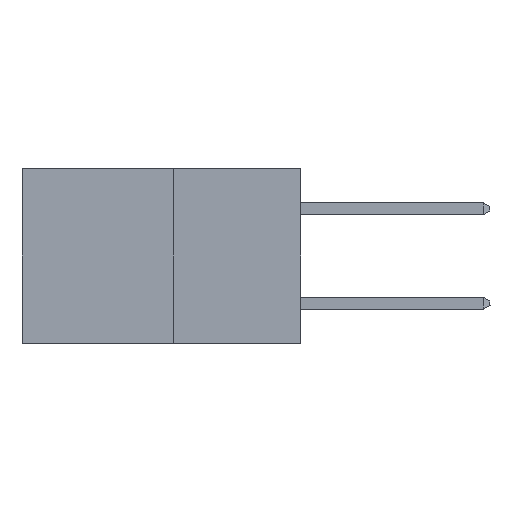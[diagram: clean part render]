
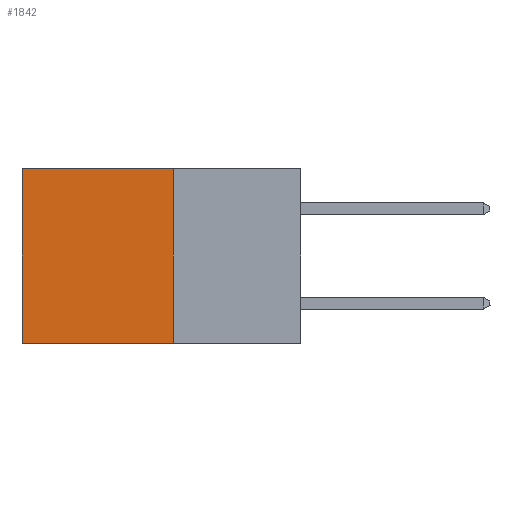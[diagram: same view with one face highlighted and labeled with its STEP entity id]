
A CAD part, left-side view. The second image highlights one B-rep face of the part: STEP entity #1842.
In plain terms, the highlighted planar face has unit normal (-1, 0, 0).
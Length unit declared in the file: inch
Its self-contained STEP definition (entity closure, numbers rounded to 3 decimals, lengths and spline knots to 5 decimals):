
#61 = CARTESIAN_POINT ( 'NONE',  ( 0.277, 0.27, -0.37 ) ) ;
#102 = CARTESIAN_POINT ( 'NONE',  ( 0.277, 0.27, -0.37 ) ) ;
#252 = DIRECTION ( 'NONE',  ( 0., 1., 0. ) ) ;
#1842 = ADVANCED_FACE ( 'NONE', ( #4763 ), #10210, .F. ) ;
#2571 = VERTEX_POINT ( 'NONE', #7368 ) ;
#2665 = EDGE_CURVE ( 'NONE', #8172, #17340, #2743, .T. ) ;
#2743 = LINE ( 'NONE', #9272, #13360 ) ;
#3216 = CARTESIAN_POINT ( 'NONE',  ( 0.277, 0.59, 0. ) ) ;
#4574 = DIRECTION ( 'NONE',  ( 1., 0., 0. ) ) ;
#4708 = ORIENTED_EDGE ( 'NONE', *, *, #6929, .T. ) ;
#4763 = FACE_OUTER_BOUND ( 'NONE', #7460, .T. ) ;
#5678 = LINE ( 'NONE', #11774, #12577 ) ;
#6779 = ORIENTED_EDGE ( 'NONE', *, *, #2665, .T. ) ;
#6929 = EDGE_CURVE ( 'NONE', #2571, #8172, #5678, .T. ) ;
#7273 = VECTOR ( 'NONE', #252, 39.37008 ) ;
#7299 = CARTESIAN_POINT ( 'NONE',  ( 0.277, 0.27, -0.37 ) ) ;
#7368 = CARTESIAN_POINT ( 'NONE',  ( 0.277, 0.27, 0. ) ) ;
#7460 = EDGE_LOOP ( 'NONE', ( #6779, #8908, #17696, #4708 ) ) ;
#7795 = DIRECTION ( 'NONE',  ( 0., 0., -1. ) ) ;
#8172 = VERTEX_POINT ( 'NONE', #3216 ) ;
#8908 = ORIENTED_EDGE ( 'NONE', *, *, #10735, .F. ) ;
#9272 = CARTESIAN_POINT ( 'NONE',  ( 0.277, 0.59, -0.37 ) ) ;
#9735 = CARTESIAN_POINT ( 'NONE',  ( 0.277, 0.59, -0.37 ) ) ;
#10210 = PLANE ( 'NONE',  #13212 ) ;
#10247 = DIRECTION ( 'NONE',  ( 0., 0., -1. ) ) ;
#10415 = DIRECTION ( 'NONE',  ( 0., 1., 0. ) ) ;
#10735 = EDGE_CURVE ( 'NONE', #15918, #17340, #14499, .T. ) ;
#11774 = CARTESIAN_POINT ( 'NONE',  ( 0.277, 0.27, 0. ) ) ;
#12577 = VECTOR ( 'NONE', #10415, 39.37008 ) ;
#12662 = DIRECTION ( 'NONE',  ( 0., 0., -1. ) ) ;
#13212 = AXIS2_PLACEMENT_3D ( 'NONE', #102, #4574, #7795 ) ;
#13360 = VECTOR ( 'NONE', #10247, 39.37008 ) ;
#13820 = VECTOR ( 'NONE', #12662, 39.37008 ) ;
#14499 = LINE ( 'NONE', #7299, #7273 ) ;
#14632 = LINE ( 'NONE', #61, #13820 ) ;
#15918 = VERTEX_POINT ( 'NONE', #16222 ) ;
#16152 = EDGE_CURVE ( 'NONE', #2571, #15918, #14632, .T. ) ;
#16222 = CARTESIAN_POINT ( 'NONE',  ( 0.277, 0.27, -0.37 ) ) ;
#17340 = VERTEX_POINT ( 'NONE', #9735 ) ;
#17696 = ORIENTED_EDGE ( 'NONE', *, *, #16152, .F. ) ;
